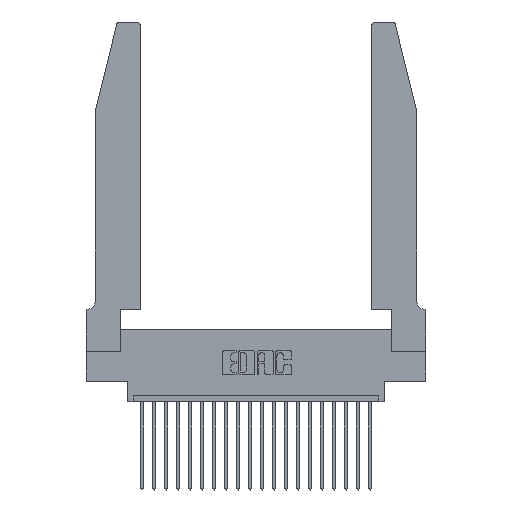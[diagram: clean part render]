
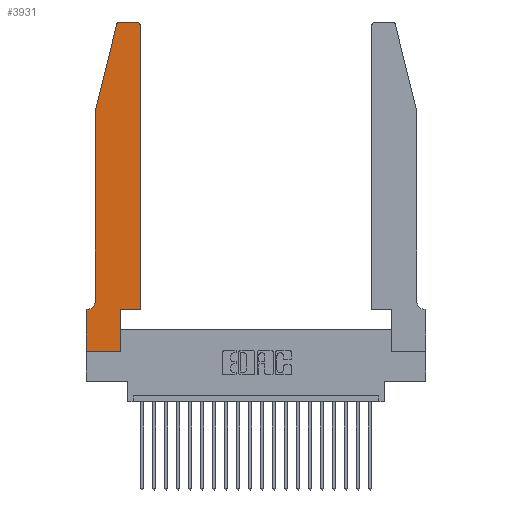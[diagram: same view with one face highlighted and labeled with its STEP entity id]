
A CAD part, top view. The second image highlights one B-rep face of the part: STEP entity #3931.
In plain terms, the highlighted planar face has unit normal (0, 0, 1).
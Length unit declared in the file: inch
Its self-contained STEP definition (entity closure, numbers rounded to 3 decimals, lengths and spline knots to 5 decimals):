
#35 = VERTEX_POINT ( 'NONE', #3524 ) ;
#144 = CIRCLE ( 'NONE', #19159, 0.03 ) ;
#174 = CARTESIAN_POINT ( 'NONE',  ( 0., 0., 0.37 ) ) ;
#179 = DIRECTION ( 'NONE',  ( 1., 0., 0. ) ) ;
#347 = VERTEX_POINT ( 'NONE', #15567 ) ;
#617 = CARTESIAN_POINT ( 'NONE',  ( 0.2865, 0.35, 0.37 ) ) ;
#1018 = CARTESIAN_POINT ( 'NONE',  ( 0.0055, 0.35, 0.37 ) ) ;
#1035 = VECTOR ( 'NONE', #1383, 39.37008 ) ;
#1049 = ORIENTED_EDGE ( 'NONE', *, *, #18998, .T. ) ;
#1334 = EDGE_CURVE ( 'NONE', #19668, #8212, #5944, .T. ) ;
#1383 = DIRECTION ( 'NONE',  ( 0., -1., 0. ) ) ;
#1533 = CARTESIAN_POINT ( 'NONE',  ( 0.0755, 0.35, 0.37 ) ) ;
#1801 = EDGE_CURVE ( 'NONE', #8212, #4462, #15284, .T. ) ;
#2073 = CIRCLE ( 'NONE', #13497, 0.07 ) ;
#2211 = LINE ( 'NONE', #13314, #4460 ) ;
#2545 = ORIENTED_EDGE ( 'NONE', *, *, #9327, .T. ) ;
#3524 = CARTESIAN_POINT ( 'NONE',  ( 0., 0.35, 0.37 ) ) ;
#3693 = ORIENTED_EDGE ( 'NONE', *, *, #8622, .T. ) ;
#3911 = DIRECTION ( 'NONE',  ( 0., 0., 1. ) ) ;
#3931 = ADVANCED_FACE ( 'NONE', ( #4395 ), #14619, .T. ) ;
#4033 = VECTOR ( 'NONE', #19147, 39.37008 ) ;
#4211 = DIRECTION ( 'NONE',  ( 1., 0., 0. ) ) ;
#4395 = FACE_OUTER_BOUND ( 'NONE', #14107, .T. ) ;
#4400 = VECTOR ( 'NONE', #22869, 39.37008 ) ;
#4460 = VECTOR ( 'NONE', #6306, 39.37008 ) ;
#4462 = VERTEX_POINT ( 'NONE', #11536 ) ;
#4586 = LINE ( 'NONE', #17442, #4033 ) ;
#4804 = CARTESIAN_POINT ( 'NONE',  ( 0., 0., 0.37 ) ) ;
#5149 = VERTEX_POINT ( 'NONE', #617 ) ;
#5282 = DIRECTION ( 'NONE',  ( 0., 1., 0. ) ) ;
#5404 = ORIENTED_EDGE ( 'NONE', *, *, #15285, .T. ) ;
#5638 = CARTESIAN_POINT ( 'NONE',  ( 0.2605, 2.75, 0.37 ) ) ;
#5944 = CIRCLE ( 'NONE', #13233, 0.03 ) ;
#6062 = EDGE_CURVE ( 'NONE', #10648, #15471, #2211, .T. ) ;
#6243 = CARTESIAN_POINT ( 'NONE',  ( 0.0055, 0.42, 0.37 ) ) ;
#6306 = DIRECTION ( 'NONE',  ( 0., 1., 0. ) ) ;
#6339 = EDGE_CURVE ( 'NONE', #18087, #347, #13580, .T. ) ;
#7008 = CARTESIAN_POINT ( 'NONE',  ( 0.284, 2.75, 0.37 ) ) ;
#7204 = VERTEX_POINT ( 'NONE', #21855 ) ;
#7441 = VECTOR ( 'NONE', #5282, 39.37008 ) ;
#7947 = VECTOR ( 'NONE', #10963, 39.37008 ) ;
#8212 = VERTEX_POINT ( 'NONE', #20409 ) ;
#8435 = ORIENTED_EDGE ( 'NONE', *, *, #20279, .T. ) ;
#8622 = EDGE_CURVE ( 'NONE', #15471, #7204, #144, .T. ) ;
#8911 = EDGE_CURVE ( 'NONE', #7204, #19668, #17357, .T. ) ;
#9174 = ORIENTED_EDGE ( 'NONE', *, *, #6062, .T. ) ;
#9327 = EDGE_CURVE ( 'NONE', #13650, #19419, #2073, .T. ) ;
#9661 = LINE ( 'NONE', #12314, #7441 ) ;
#10460 = CARTESIAN_POINT ( 'NONE',  ( 0.0755, 2., 0.37 ) ) ;
#10648 = VERTEX_POINT ( 'NONE', #21085 ) ;
#10825 = DIRECTION ( 'NONE',  ( 0., 0., 1. ) ) ;
#10896 = ORIENTED_EDGE ( 'NONE', *, *, #22071, .T. ) ;
#10963 = DIRECTION ( 'NONE',  ( -1., 0., 0. ) ) ;
#11536 = CARTESIAN_POINT ( 'NONE',  ( 0.0755, 2., 0.37 ) ) ;
#11541 = DIRECTION ( 'NONE',  ( 0., 0., -1. ) ) ;
#11623 = DIRECTION ( 'NONE',  ( -1., 0., 0. ) ) ;
#12314 = CARTESIAN_POINT ( 'NONE',  ( 0.2865, 0.35, 0.37 ) ) ;
#12328 = LINE ( 'NONE', #4804, #21110 ) ;
#12589 = DIRECTION ( 'NONE',  ( 1., 0., 0. ) ) ;
#12778 = DIRECTION ( 'NONE',  ( 1., 0., 0. ) ) ;
#12855 = CARTESIAN_POINT ( 'NONE',  ( 0.4205, 2.72, 0.37 ) ) ;
#13233 = AXIS2_PLACEMENT_3D ( 'NONE', #19646, #10825, #179 ) ;
#13314 = CARTESIAN_POINT ( 'NONE',  ( 0.4505, 0.35, 0.37 ) ) ;
#13497 = AXIS2_PLACEMENT_3D ( 'NONE', #6243, #11541, #11623 ) ;
#13580 = LINE ( 'NONE', #174, #18294 ) ;
#13650 = VERTEX_POINT ( 'NONE', #22160 ) ;
#13897 = DIRECTION ( 'NONE',  ( 0., -1., 0. ) ) ;
#14107 = EDGE_LOOP ( 'NONE', ( #19638, #20333, #20280, #8435, #2545, #16159, #1049, #16129, #5404, #10896, #9174, #3693 ) ) ;
#14619 = PLANE ( 'NONE',  #20571 ) ;
#15001 = DIRECTION ( 'NONE',  ( -0.239, -0.971, 0. ) ) ;
#15167 = LINE ( 'NONE', #1533, #4400 ) ;
#15180 = EDGE_CURVE ( 'NONE', #19419, #35, #15167, .T. ) ;
#15284 = LINE ( 'NONE', #18293, #21632 ) ;
#15285 = EDGE_CURVE ( 'NONE', #347, #5149, #9661, .T. ) ;
#15471 = VERTEX_POINT ( 'NONE', #16462 ) ;
#15567 = CARTESIAN_POINT ( 'NONE',  ( 0.2865, 0., 0.37 ) ) ;
#16129 = ORIENTED_EDGE ( 'NONE', *, *, #6339, .T. ) ;
#16159 = ORIENTED_EDGE ( 'NONE', *, *, #15180, .T. ) ;
#16462 = CARTESIAN_POINT ( 'NONE',  ( 0.4505, 2.72, 0.37 ) ) ;
#16491 = CARTESIAN_POINT ( 'NONE',  ( 0., 0.35, 0.37 ) ) ;
#17357 = LINE ( 'NONE', #5638, #7947 ) ;
#17442 = CARTESIAN_POINT ( 'NONE',  ( 0.4505, 0.35, 0.37 ) ) ;
#18087 = VERTEX_POINT ( 'NONE', #21804 ) ;
#18293 = CARTESIAN_POINT ( 'NONE',  ( 0.0755, 2., 0.37 ) ) ;
#18294 = VECTOR ( 'NONE', #12589, 39.37008 ) ;
#18998 = EDGE_CURVE ( 'NONE', #35, #18087, #12328, .T. ) ;
#19147 = DIRECTION ( 'NONE',  ( 1., 0., 0. ) ) ;
#19159 = AXIS2_PLACEMENT_3D ( 'NONE', #12855, #21894, #4211 ) ;
#19419 = VERTEX_POINT ( 'NONE', #1018 ) ;
#19638 = ORIENTED_EDGE ( 'NONE', *, *, #8911, .T. ) ;
#19646 = CARTESIAN_POINT ( 'NONE',  ( 0.284, 2.72, 0.37 ) ) ;
#19668 = VERTEX_POINT ( 'NONE', #7008 ) ;
#20279 = EDGE_CURVE ( 'NONE', #4462, #13650, #20709, .T. ) ;
#20280 = ORIENTED_EDGE ( 'NONE', *, *, #1801, .T. ) ;
#20333 = ORIENTED_EDGE ( 'NONE', *, *, #1334, .T. ) ;
#20409 = CARTESIAN_POINT ( 'NONE',  ( 0.25487, 2.72718, 0.37 ) ) ;
#20571 = AXIS2_PLACEMENT_3D ( 'NONE', #16491, #3911, #12778 ) ;
#20709 = LINE ( 'NONE', #10460, #1035 ) ;
#21085 = CARTESIAN_POINT ( 'NONE',  ( 0.4505, 0.35, 0.37 ) ) ;
#21110 = VECTOR ( 'NONE', #13897, 39.37008 ) ;
#21632 = VECTOR ( 'NONE', #15001, 39.37008 ) ;
#21804 = CARTESIAN_POINT ( 'NONE',  ( 0., 0., 0.37 ) ) ;
#21855 = CARTESIAN_POINT ( 'NONE',  ( 0.4205, 2.75, 0.37 ) ) ;
#21894 = DIRECTION ( 'NONE',  ( 0., 0., 1. ) ) ;
#22071 = EDGE_CURVE ( 'NONE', #5149, #10648, #4586, .T. ) ;
#22160 = CARTESIAN_POINT ( 'NONE',  ( 0.0755, 0.42, 0.37 ) ) ;
#22869 = DIRECTION ( 'NONE',  ( -1., 0., 0. ) ) ;
